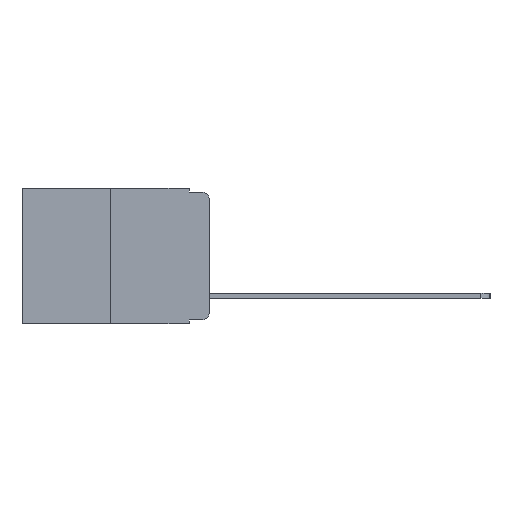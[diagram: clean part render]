
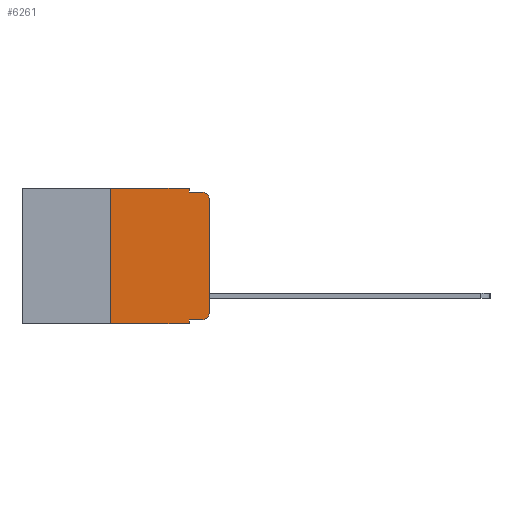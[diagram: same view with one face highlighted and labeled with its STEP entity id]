
A CAD part, left-side view. The second image highlights one B-rep face of the part: STEP entity #6261.
In plain terms, the highlighted planar face has unit normal (-1, 0, 0).
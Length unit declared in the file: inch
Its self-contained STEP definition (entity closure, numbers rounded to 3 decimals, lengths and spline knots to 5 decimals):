
#285 = VERTEX_POINT ( 'NONE', #4013 ) ;
#385 = ORIENTED_EDGE ( 'NONE', *, *, #10582, .F. ) ;
#410 = DIRECTION ( 'NONE',  ( 0., 0., -1. ) ) ;
#487 = EDGE_CURVE ( 'NONE', #285, #6591, #8816, .T. ) ;
#570 = ORIENTED_EDGE ( 'NONE', *, *, #6384, .T. ) ;
#666 = EDGE_LOOP ( 'NONE', ( #6935, #889, #1813, #11111, #385, #4904, #570, #8856, #9125, #7898 ) ) ;
#870 = CARTESIAN_POINT ( 'NONE',  ( 0., 0.473, 0. ) ) ;
#877 = AXIS2_PLACEMENT_3D ( 'NONE', #9354, #4182, #10227 ) ;
#889 = ORIENTED_EDGE ( 'NONE', *, *, #3069, .T. ) ;
#1089 = VERTEX_POINT ( 'NONE', #3571 ) ;
#1109 = VERTEX_POINT ( 'NONE', #1461 ) ;
#1113 = CIRCLE ( 'NONE', #877, 0.02 ) ;
#1138 = DIRECTION ( 'NONE',  ( 1., 0., 0. ) ) ;
#1188 = EDGE_CURVE ( 'NONE', #2026, #4310, #7363, .T. ) ;
#1253 = CARTESIAN_POINT ( 'NONE',  ( 0., 0.473, 0. ) ) ;
#1272 = LINE ( 'NONE', #11332, #10123 ) ;
#1350 = PLANE ( 'NONE',  #9926 ) ;
#1461 = CARTESIAN_POINT ( 'NONE',  ( 0., 0.051, 0. ) ) ;
#1621 = DIRECTION ( 'NONE',  ( 0., 0., 1. ) ) ;
#1656 = CARTESIAN_POINT ( 'NONE',  ( 0., 0.25, 0. ) ) ;
#1813 = ORIENTED_EDGE ( 'NONE', *, *, #2461, .F. ) ;
#1838 = EDGE_CURVE ( 'NONE', #1109, #1978, #7084, .T. ) ;
#1978 = VERTEX_POINT ( 'NONE', #8893 ) ;
#2026 = VERTEX_POINT ( 'NONE', #3521 ) ;
#2261 = VECTOR ( 'NONE', #7950, 39.37008 ) ;
#2357 = CARTESIAN_POINT ( 'NONE',  ( 0., 0.02, -0.03 ) ) ;
#2461 = EDGE_CURVE ( 'NONE', #1978, #5460, #11517, .T. ) ;
#2942 = CARTESIAN_POINT ( 'NONE',  ( 0., 0.051, -0.343 ) ) ;
#3034 = FACE_OUTER_BOUND ( 'NONE', #666, .T. ) ;
#3069 = EDGE_CURVE ( 'NONE', #1089, #5460, #10976, .T. ) ;
#3521 = CARTESIAN_POINT ( 'NONE',  ( 0., 0.25, -0.343 ) ) ;
#3571 = CARTESIAN_POINT ( 'NONE',  ( 0., 0., -0.03 ) ) ;
#3674 = EDGE_CURVE ( 'NONE', #11141, #1089, #8139, .T. ) ;
#4013 = CARTESIAN_POINT ( 'NONE',  ( 0., 0.051, -0.333 ) ) ;
#4085 = DIRECTION ( 'NONE',  ( -1., 0., 0. ) ) ;
#4182 = DIRECTION ( 'NONE',  ( -1., 0., 0. ) ) ;
#4215 = VECTOR ( 'NONE', #5701, 39.37008 ) ;
#4264 = CARTESIAN_POINT ( 'NONE',  ( 0., 0.051, 0. ) ) ;
#4310 = VERTEX_POINT ( 'NONE', #11221 ) ;
#4570 = DIRECTION ( 'NONE',  ( 0., -1., 0. ) ) ;
#4679 = VECTOR ( 'NONE', #4570, 39.37008 ) ;
#4904 = ORIENTED_EDGE ( 'NONE', *, *, #1188, .F. ) ;
#5047 = VECTOR ( 'NONE', #1621, 39.37008 ) ;
#5460 = VERTEX_POINT ( 'NONE', #8135 ) ;
#5701 = DIRECTION ( 'NONE',  ( 0., 0., -1. ) ) ;
#6261 = ADVANCED_FACE ( 'NONE', ( #3034 ), #1350, .F. ) ;
#6354 = CARTESIAN_POINT ( 'NONE',  ( 0., 0.051, -0.333 ) ) ;
#6384 = EDGE_CURVE ( 'NONE', #2026, #6591, #1272, .T. ) ;
#6591 = VERTEX_POINT ( 'NONE', #2942 ) ;
#6755 = VERTEX_POINT ( 'NONE', #8850 ) ;
#6935 = ORIENTED_EDGE ( 'NONE', *, *, #3674, .T. ) ;
#6995 = LINE ( 'NONE', #870, #4679 ) ;
#7084 = LINE ( 'NONE', #9179, #7885 ) ;
#7363 = LINE ( 'NONE', #1656, #5047 ) ;
#7425 = DIRECTION ( 'NONE',  ( 0., -1., 0. ) ) ;
#7866 = VECTOR ( 'NONE', #10052, 39.37008 ) ;
#7885 = VECTOR ( 'NONE', #9338, 39.37008 ) ;
#7898 = ORIENTED_EDGE ( 'NONE', *, *, #10295, .T. ) ;
#7950 = DIRECTION ( 'NONE',  ( 0., -1., 0. ) ) ;
#8077 = DIRECTION ( 'NONE',  ( 0., -1., 0. ) ) ;
#8135 = CARTESIAN_POINT ( 'NONE',  ( 0., 0.02, -0.01 ) ) ;
#8139 = LINE ( 'NONE', #10019, #7866 ) ;
#8145 = AXIS2_PLACEMENT_3D ( 'NONE', #2357, #4085, #11273 ) ;
#8280 = CARTESIAN_POINT ( 'NONE',  ( 0., 0.051, -0.01 ) ) ;
#8331 = VECTOR ( 'NONE', #8077, 39.37008 ) ;
#8816 = LINE ( 'NONE', #4264, #4215 ) ;
#8850 = CARTESIAN_POINT ( 'NONE',  ( 0., 0.02, -0.333 ) ) ;
#8856 = ORIENTED_EDGE ( 'NONE', *, *, #487, .F. ) ;
#8893 = CARTESIAN_POINT ( 'NONE',  ( 0., 0.051, -0.01 ) ) ;
#9125 = ORIENTED_EDGE ( 'NONE', *, *, #11417, .T. ) ;
#9179 = CARTESIAN_POINT ( 'NONE',  ( 0., 0.051, 0. ) ) ;
#9338 = DIRECTION ( 'NONE',  ( 0., 0., -1. ) ) ;
#9354 = CARTESIAN_POINT ( 'NONE',  ( 0., 0.02, -0.313 ) ) ;
#9542 = CARTESIAN_POINT ( 'NONE',  ( 0., 0., -0.313 ) ) ;
#9926 = AXIS2_PLACEMENT_3D ( 'NONE', #1253, #1138, #410 ) ;
#10019 = CARTESIAN_POINT ( 'NONE',  ( 0., 0., 0. ) ) ;
#10052 = DIRECTION ( 'NONE',  ( 0., 0., 1. ) ) ;
#10123 = VECTOR ( 'NONE', #7425, 39.37008 ) ;
#10227 = DIRECTION ( 'NONE',  ( 0., 0., -1. ) ) ;
#10295 = EDGE_CURVE ( 'NONE', #6755, #11141, #1113, .T. ) ;
#10582 = EDGE_CURVE ( 'NONE', #4310, #1109, #6995, .T. ) ;
#10609 = LINE ( 'NONE', #6354, #8331 ) ;
#10976 = CIRCLE ( 'NONE', #8145, 0.02 ) ;
#11111 = ORIENTED_EDGE ( 'NONE', *, *, #1838, .F. ) ;
#11141 = VERTEX_POINT ( 'NONE', #9542 ) ;
#11221 = CARTESIAN_POINT ( 'NONE',  ( 0., 0.25, 0. ) ) ;
#11273 = DIRECTION ( 'NONE',  ( 0., 0., -1. ) ) ;
#11332 = CARTESIAN_POINT ( 'NONE',  ( 0., 0.473, -0.343 ) ) ;
#11417 = EDGE_CURVE ( 'NONE', #285, #6755, #10609, .T. ) ;
#11517 = LINE ( 'NONE', #8280, #2261 ) ;
